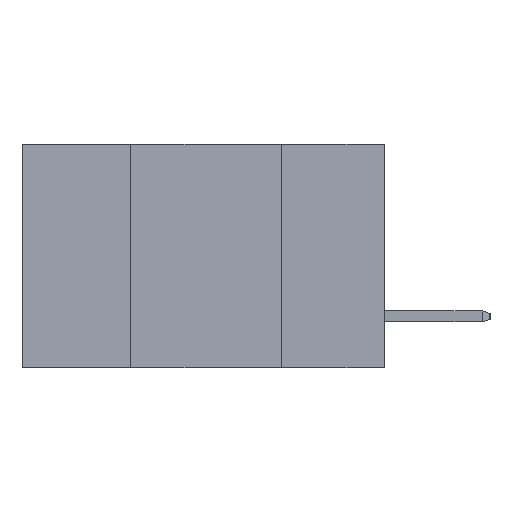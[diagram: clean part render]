
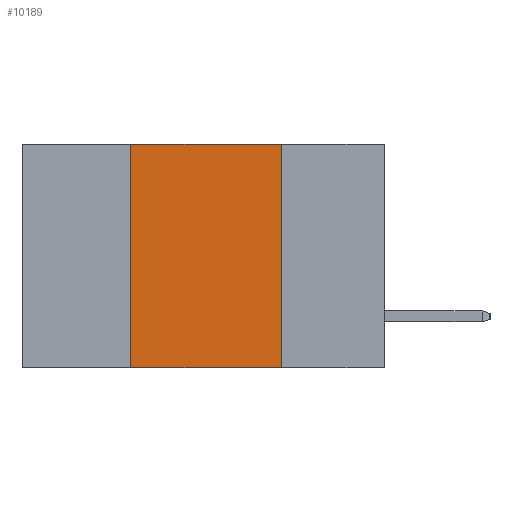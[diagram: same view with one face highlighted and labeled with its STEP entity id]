
A CAD part, left-side view. The second image highlights one B-rep face of the part: STEP entity #10189.
In plain terms, the highlighted planar face has unit normal (-1, 0, 0).
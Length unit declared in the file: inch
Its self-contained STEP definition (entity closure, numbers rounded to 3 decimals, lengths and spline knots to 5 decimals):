
#324 = VERTEX_POINT ( 'NONE', #7200 ) ;
#1378 = EDGE_CURVE ( 'NONE', #20709, #324, #14548, .T. ) ;
#2531 = LINE ( 'NONE', #18264, #19295 ) ;
#2661 = EDGE_LOOP ( 'NONE', ( #7142, #9575, #12957, #5812 ) ) ;
#4931 = EDGE_CURVE ( 'NONE', #324, #15692, #9562, .T. ) ;
#5028 = VECTOR ( 'NONE', #8817, 39.37008 ) ;
#5554 = VECTOR ( 'NONE', #12658, 39.37008 ) ;
#5812 = ORIENTED_EDGE ( 'NONE', *, *, #15500, .T. ) ;
#7142 = ORIENTED_EDGE ( 'NONE', *, *, #4931, .F. ) ;
#7200 = CARTESIAN_POINT ( 'NONE',  ( 0., 0.17, 0. ) ) ;
#8419 = CARTESIAN_POINT ( 'NONE',  ( 0., 0.17, -0.37 ) ) ;
#8817 = DIRECTION ( 'NONE',  ( 0., 0., -1. ) ) ;
#8995 = CARTESIAN_POINT ( 'NONE',  ( 0., 0.17, -0.37 ) ) ;
#9109 = VERTEX_POINT ( 'NONE', #17598 ) ;
#9562 = LINE ( 'NONE', #8419, #5028 ) ;
#9575 = ORIENTED_EDGE ( 'NONE', *, *, #1378, .F. ) ;
#9596 = CARTESIAN_POINT ( 'NONE',  ( 0., 0.42, 0. ) ) ;
#10189 = ADVANCED_FACE ( 'NONE', ( #16245 ), #17214, .F. ) ;
#10489 = EDGE_CURVE ( 'NONE', #9109, #20709, #19279, .T. ) ;
#11005 = CARTESIAN_POINT ( 'NONE',  ( 0., 0.6, 0. ) ) ;
#12658 = DIRECTION ( 'NONE',  ( 0., -1., 0. ) ) ;
#12957 = ORIENTED_EDGE ( 'NONE', *, *, #10489, .F. ) ;
#13610 = CARTESIAN_POINT ( 'NONE',  ( 0., 0.42, -0.37 ) ) ;
#13634 = DIRECTION ( 'NONE',  ( 0., 0., 1. ) ) ;
#14548 = LINE ( 'NONE', #11005, #5554 ) ;
#14925 = VECTOR ( 'NONE', #13634, 39.37008 ) ;
#15500 = EDGE_CURVE ( 'NONE', #9109, #15692, #2531, .T. ) ;
#15602 = AXIS2_PLACEMENT_3D ( 'NONE', #17124, #17117, #17101 ) ;
#15692 = VERTEX_POINT ( 'NONE', #8995 ) ;
#16245 = FACE_OUTER_BOUND ( 'NONE', #2661, .T. ) ;
#17101 = DIRECTION ( 'NONE',  ( 0., 0., -1. ) ) ;
#17117 = DIRECTION ( 'NONE',  ( 1., 0., 0. ) ) ;
#17124 = CARTESIAN_POINT ( 'NONE',  ( 0., 0.6, 0. ) ) ;
#17214 = PLANE ( 'NONE',  #15602 ) ;
#17598 = CARTESIAN_POINT ( 'NONE',  ( 0., 0.42, -0.37 ) ) ;
#18264 = CARTESIAN_POINT ( 'NONE',  ( 0., 0.6, -0.37 ) ) ;
#19279 = LINE ( 'NONE', #13610, #14925 ) ;
#19295 = VECTOR ( 'NONE', #20179, 39.37008 ) ;
#20179 = DIRECTION ( 'NONE',  ( 0., -1., 0. ) ) ;
#20709 = VERTEX_POINT ( 'NONE', #9596 ) ;
